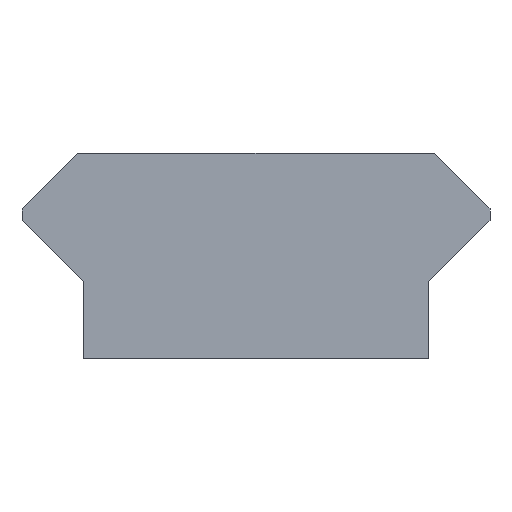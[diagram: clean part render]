
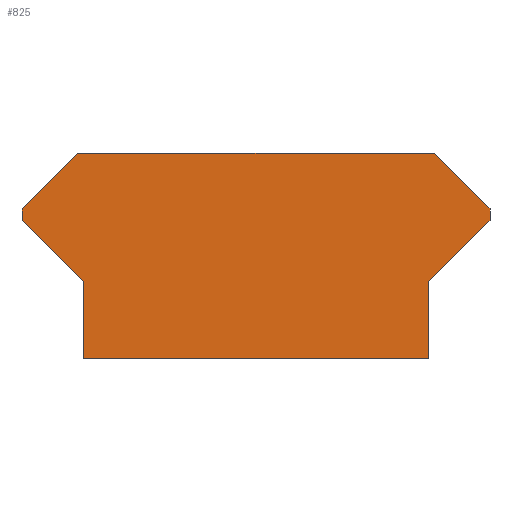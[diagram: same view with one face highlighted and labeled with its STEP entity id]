
A CAD part, front view. The second image highlights one B-rep face of the part: STEP entity #825.
In plain terms, the highlighted planar face has unit normal (0, -1, 0).
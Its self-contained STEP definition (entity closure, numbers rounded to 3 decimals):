
#19=FACE_OUTER_BOUND('',#61,.T.);
#61=EDGE_LOOP('',(#575,#576,#577,#578,#579,#580,#581,#582,#583,#584));
#99=LINE('',#1129,#219);
#103=LINE('',#1137,#223);
#106=LINE('',#1143,#226);
#129=LINE('',#1189,#249);
#132=LINE('',#1195,#252);
#133=LINE('',#1197,#253);
#134=LINE('',#1199,#254);
#135=LINE('',#1201,#255);
#136=LINE('',#1203,#256);
#137=LINE('',#1204,#257);
#219=VECTOR('',#923,10.);
#223=VECTOR('',#929,10.);
#226=VECTOR('',#934,10.);
#249=VECTOR('',#959,10.);
#252=VECTOR('',#964,10.);
#253=VECTOR('',#965,10.);
#254=VECTOR('',#966,10.);
#255=VECTOR('',#967,10.);
#256=VECTOR('',#968,10.);
#257=VECTOR('',#969,10.);
#339=VERTEX_POINT('',#1127);
#340=VERTEX_POINT('',#1128);
#343=VERTEX_POINT('',#1136);
#345=VERTEX_POINT('',#1142);
#367=VERTEX_POINT('',#1188);
#369=VERTEX_POINT('',#1194);
#370=VERTEX_POINT('',#1196);
#371=VERTEX_POINT('',#1198);
#372=VERTEX_POINT('',#1200);
#373=VERTEX_POINT('',#1202);
#419=EDGE_CURVE('',#339,#340,#99,.T.);
#423=EDGE_CURVE('',#340,#343,#103,.T.);
#426=EDGE_CURVE('',#343,#345,#106,.T.);
#449=EDGE_CURVE('',#367,#339,#129,.T.);
#452=EDGE_CURVE('',#369,#345,#132,.T.);
#453=EDGE_CURVE('',#370,#369,#133,.T.);
#454=EDGE_CURVE('',#371,#370,#134,.T.);
#455=EDGE_CURVE('',#371,#372,#135,.T.);
#456=EDGE_CURVE('',#372,#373,#136,.T.);
#457=EDGE_CURVE('',#373,#367,#137,.T.);
#575=ORIENTED_EDGE('',*,*,#426,.T.);
#576=ORIENTED_EDGE('',*,*,#452,.F.);
#577=ORIENTED_EDGE('',*,*,#453,.F.);
#578=ORIENTED_EDGE('',*,*,#454,.F.);
#579=ORIENTED_EDGE('',*,*,#455,.T.);
#580=ORIENTED_EDGE('',*,*,#456,.T.);
#581=ORIENTED_EDGE('',*,*,#457,.T.);
#582=ORIENTED_EDGE('',*,*,#449,.T.);
#583=ORIENTED_EDGE('',*,*,#419,.T.);
#584=ORIENTED_EDGE('',*,*,#423,.T.);
#783=PLANE('',#881);
#825=ADVANCED_FACE('',(#19),#783,.F.);
#881=AXIS2_PLACEMENT_3D('',#1193,#962,#963);
#923=DIRECTION('',(0.,0.,1.));
#929=DIRECTION('',(0.707,0.,0.707));
#934=DIRECTION('',(0.,0.,1.));
#959=DIRECTION('',(1.,0.,0.));
#962=DIRECTION('center_axis',(0.,1.,0.));
#963=DIRECTION('ref_axis',(0.,0.,1.));
#964=DIRECTION('',(0.707,0.,-0.707));
#965=DIRECTION('',(1.,0.,0.));
#966=DIRECTION('',(0.707,0.,0.707));
#967=DIRECTION('',(0.,0.,-1.));
#968=DIRECTION('',(0.707,0.,-0.707));
#969=DIRECTION('',(0.,0.,-1.));
#1127=CARTESIAN_POINT('',(7.836,27.653,-22.403));
#1128=CARTESIAN_POINT('',(7.836,27.653,-18.91));
#1129=CARTESIAN_POINT('',(7.836,27.653,-18.205));
#1136=CARTESIAN_POINT('',(10.605,27.653,-16.142));
#1137=CARTESIAN_POINT('',(7.553,27.653,-19.193));
#1142=CARTESIAN_POINT('',(10.605,27.653,-15.608));
#1143=CARTESIAN_POINT('',(10.605,27.653,-16.675));
#1188=CARTESIAN_POINT('',(-7.836,27.653,-22.403));
#1189=CARTESIAN_POINT('',(-3.918,27.653,-22.403));
#1193=CARTESIAN_POINT('Origin',(-10.605,27.653,-16.078));
#1194=CARTESIAN_POINT('',(8.077,27.653,-13.081));
#1195=CARTESIAN_POINT('',(4.867,27.653,-9.871));
#1196=CARTESIAN_POINT('',(-8.077,27.653,-13.081));
#1197=CARTESIAN_POINT('',(-9.341,27.653,-13.081));
#1198=CARTESIAN_POINT('',(-10.605,27.653,-15.608));
#1199=CARTESIAN_POINT('',(-10.17,27.653,-15.173));
#1200=CARTESIAN_POINT('',(-10.605,27.653,-16.142));
#1201=CARTESIAN_POINT('',(-10.605,27.653,-16.675));
#1202=CARTESIAN_POINT('',(-7.836,27.653,-18.91));
#1203=CARTESIAN_POINT('',(-7.001,27.653,-19.745));
#1204=CARTESIAN_POINT('',(-7.836,27.653,-18.205));
